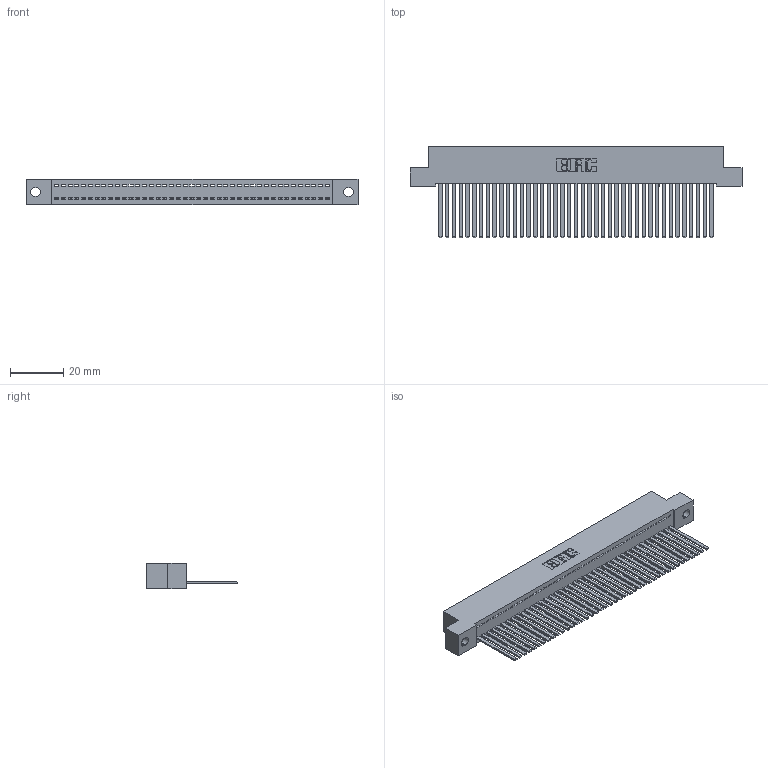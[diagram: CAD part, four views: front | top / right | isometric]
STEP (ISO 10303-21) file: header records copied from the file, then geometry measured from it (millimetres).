
FILE_DESCRIPTION (( 'STEP AP203' ), '1' );
FILE_NAME ('342-041-544-102.STEP', '2019-10-02T17:27:44', ( '' ), ( '' ), 'SwSTEP 2.0', 'SolidWorks 2016', '' );
FILE_SCHEMA (( 'CONFIG_CONTROL_DESIGN' ));
Length unit declared in the file: inch
Products named in the file (3): 342-041-544-102; 342 Part_.128 Slot; 345-292-001_345-293-144
Assembly tree (42 placements, depth 2):
  342-041-544-102
    342 Part_.128 Slot
    345-292-001_345-293-144  x41
Bounding box: 124.46 x 34.3 x 9.4 mm (x, y, z)
Volume: 11331.7 mm3; surface area: 17732.4 mm2
Topology: 42 solids, 42 shells, 2246 faces, 6789 edges, 4470 vertices
Faces by surface type: plane 1628, cylinder 618
Entity records: 25013 total; most frequent: CARTESIAN_POINT 4321, ORIENTED_EDGE 4298, DIRECTION 3643, EDGE_CURVE 2149, LINE 2025, VECTOR 2025, VERTEX_POINT 1430, AXIS2_PLACEMENT_3D 809
